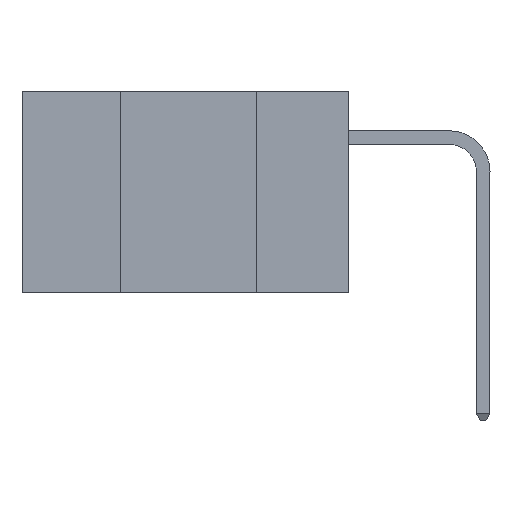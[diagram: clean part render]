
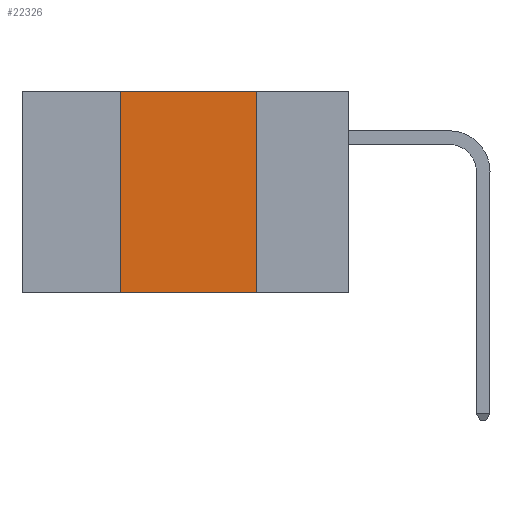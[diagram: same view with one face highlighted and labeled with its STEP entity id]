
A CAD part, left-side view. The second image highlights one B-rep face of the part: STEP entity #22326.
In plain terms, the highlighted planar face has unit normal (-1, 0, 0).
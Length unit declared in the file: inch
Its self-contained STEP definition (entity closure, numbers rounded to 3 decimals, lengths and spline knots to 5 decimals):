
#101 = LINE ( 'NONE', #31851, #16474 ) ;
#2246 = CARTESIAN_POINT ( 'NONE',  ( 0., 0.42, 0. ) ) ;
#3609 = ORIENTED_EDGE ( 'NONE', *, *, #4680, .F. ) ;
#4680 = EDGE_CURVE ( 'NONE', #16041, #27597, #11918, .T. ) ;
#4929 = EDGE_LOOP ( 'NONE', ( #17765, #3609, #23558, #20710 ) ) ;
#6827 = DIRECTION ( 'NONE',  ( 0., 0., -1. ) ) ;
#8021 = AXIS2_PLACEMENT_3D ( 'NONE', #20063, #34022, #6827 ) ;
#8129 = CARTESIAN_POINT ( 'NONE',  ( 0., 0.42, 0. ) ) ;
#10039 = FACE_OUTER_BOUND ( 'NONE', #4929, .T. ) ;
#10246 = CARTESIAN_POINT ( 'NONE',  ( 0., 0.42, -0.37 ) ) ;
#10827 = EDGE_CURVE ( 'NONE', #25770, #16041, #20463, .T. ) ;
#10871 = DIRECTION ( 'NONE',  ( 0., 0., -1. ) ) ;
#11734 = CARTESIAN_POINT ( 'NONE',  ( 0., 0.17, -0.37 ) ) ;
#11918 = LINE ( 'NONE', #25716, #30364 ) ;
#14583 = DIRECTION ( 'NONE',  ( 0., -1., 0. ) ) ;
#16041 = VERTEX_POINT ( 'NONE', #8129 ) ;
#16302 = CARTESIAN_POINT ( 'NONE',  ( 0., 0.17, 0. ) ) ;
#16420 = DIRECTION ( 'NONE',  ( 0., 0., 1. ) ) ;
#16474 = VECTOR ( 'NONE', #14583, 39.37008 ) ;
#17182 = EDGE_CURVE ( 'NONE', #27597, #21158, #20553, .T. ) ;
#17765 = ORIENTED_EDGE ( 'NONE', *, *, #17182, .F. ) ;
#20063 = CARTESIAN_POINT ( 'NONE',  ( 0., 0.6, 0. ) ) ;
#20463 = LINE ( 'NONE', #2246, #29007 ) ;
#20553 = LINE ( 'NONE', #16302, #29118 ) ;
#20710 = ORIENTED_EDGE ( 'NONE', *, *, #34971, .T. ) ;
#21158 = VERTEX_POINT ( 'NONE', #11734 ) ;
#22326 = ADVANCED_FACE ( 'NONE', ( #10039 ), #23318, .F. ) ;
#23318 = PLANE ( 'NONE',  #8021 ) ;
#23558 = ORIENTED_EDGE ( 'NONE', *, *, #10827, .F. ) ;
#25716 = CARTESIAN_POINT ( 'NONE',  ( 0., 0.6, 0. ) ) ;
#25770 = VERTEX_POINT ( 'NONE', #10246 ) ;
#26559 = CARTESIAN_POINT ( 'NONE',  ( 0., 0.17, 0. ) ) ;
#27597 = VERTEX_POINT ( 'NONE', #26559 ) ;
#29007 = VECTOR ( 'NONE', #16420, 39.37008 ) ;
#29118 = VECTOR ( 'NONE', #10871, 39.37008 ) ;
#30364 = VECTOR ( 'NONE', #34047, 39.37008 ) ;
#31851 = CARTESIAN_POINT ( 'NONE',  ( 0., 0.6, -0.37 ) ) ;
#34022 = DIRECTION ( 'NONE',  ( 1., 0., 0. ) ) ;
#34047 = DIRECTION ( 'NONE',  ( 0., -1., 0. ) ) ;
#34971 = EDGE_CURVE ( 'NONE', #25770, #21158, #101, .T. ) ;
